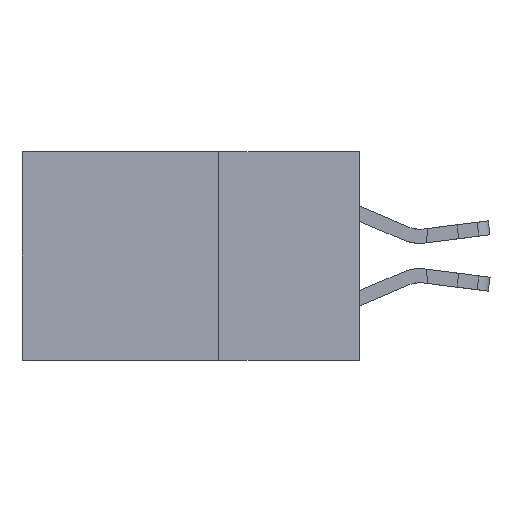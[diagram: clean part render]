
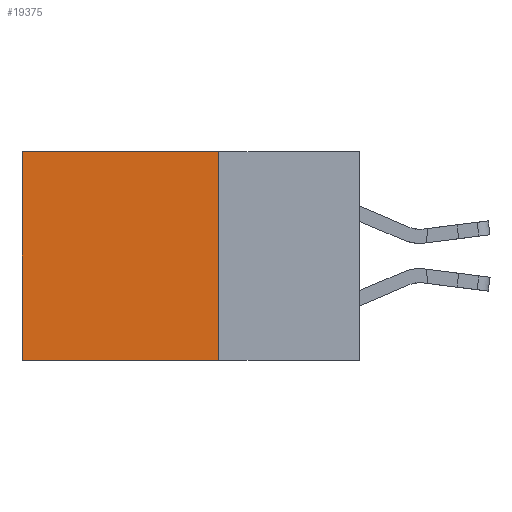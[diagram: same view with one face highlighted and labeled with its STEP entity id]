
A CAD part, left-side view. The second image highlights one B-rep face of the part: STEP entity #19375.
In plain terms, the highlighted planar face has unit normal (-1, 0, 0).
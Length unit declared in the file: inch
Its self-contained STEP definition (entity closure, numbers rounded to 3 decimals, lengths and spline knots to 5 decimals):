
#25 = DIRECTION ( 'NONE',  ( 0., 0., -1. ) ) ;
#380 = EDGE_LOOP ( 'NONE', ( #5712, #18818, #11162, #16852 ) ) ;
#696 = VERTEX_POINT ( 'NONE', #4495 ) ;
#1510 = CARTESIAN_POINT ( 'NONE',  ( 0.2875, 0.6, -0.37 ) ) ;
#1590 = VERTEX_POINT ( 'NONE', #15458 ) ;
#4495 = CARTESIAN_POINT ( 'NONE',  ( 0.2875, 0.6, 0. ) ) ;
#5712 = ORIENTED_EDGE ( 'NONE', *, *, #28996, .T. ) ;
#6958 = EDGE_CURVE ( 'NONE', #15104, #1590, #29315, .T. ) ;
#7219 = CARTESIAN_POINT ( 'NONE',  ( 0.2875, 0.25, 0. ) ) ;
#7956 = EDGE_CURVE ( 'NONE', #1590, #23263, #11143, .T. ) ;
#9036 = VECTOR ( 'NONE', #22321, 39.37008 ) ;
#9508 = DIRECTION ( 'NONE',  ( 0., 0., -1. ) ) ;
#11143 = LINE ( 'NONE', #17232, #27171 ) ;
#11162 = ORIENTED_EDGE ( 'NONE', *, *, #6958, .F. ) ;
#12771 = DIRECTION ( 'NONE',  ( 0., 1., 0. ) ) ;
#13153 = VECTOR ( 'NONE', #25, 39.37008 ) ;
#14085 = DIRECTION ( 'NONE',  ( 1., 0., 0. ) ) ;
#15104 = VERTEX_POINT ( 'NONE', #16599 ) ;
#15458 = CARTESIAN_POINT ( 'NONE',  ( 0.2875, 0.25, -0.37 ) ) ;
#16255 = PLANE ( 'NONE',  #16635 ) ;
#16283 = CARTESIAN_POINT ( 'NONE',  ( 0.2875, 0.6, 0. ) ) ;
#16599 = CARTESIAN_POINT ( 'NONE',  ( 0.2875, 0.25, 0. ) ) ;
#16635 = AXIS2_PLACEMENT_3D ( 'NONE', #7219, #14085, #9508 ) ;
#16852 = ORIENTED_EDGE ( 'NONE', *, *, #24436, .T. ) ;
#17232 = CARTESIAN_POINT ( 'NONE',  ( 0.2875, 0.25, -0.37 ) ) ;
#17299 = DIRECTION ( 'NONE',  ( 0., 0., -1. ) ) ;
#17383 = CARTESIAN_POINT ( 'NONE',  ( 0.2875, 0.25, 0. ) ) ;
#18818 = ORIENTED_EDGE ( 'NONE', *, *, #7956, .F. ) ;
#19375 = ADVANCED_FACE ( 'NONE', ( #22557 ), #16255, .F. ) ;
#20821 = LINE ( 'NONE', #17383, #9036 ) ;
#22321 = DIRECTION ( 'NONE',  ( 0., 1., 0. ) ) ;
#22557 = FACE_OUTER_BOUND ( 'NONE', #380, .T. ) ;
#22587 = VECTOR ( 'NONE', #17299, 39.37008 ) ;
#23263 = VERTEX_POINT ( 'NONE', #1510 ) ;
#23513 = LINE ( 'NONE', #16283, #13153 ) ;
#24019 = CARTESIAN_POINT ( 'NONE',  ( 0.2875, 0.25, 0. ) ) ;
#24436 = EDGE_CURVE ( 'NONE', #15104, #696, #20821, .T. ) ;
#27171 = VECTOR ( 'NONE', #12771, 39.37008 ) ;
#28996 = EDGE_CURVE ( 'NONE', #696, #23263, #23513, .T. ) ;
#29315 = LINE ( 'NONE', #24019, #22587 ) ;
